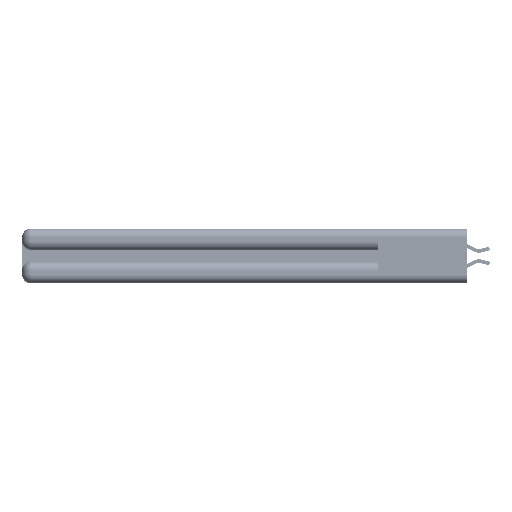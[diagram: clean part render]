
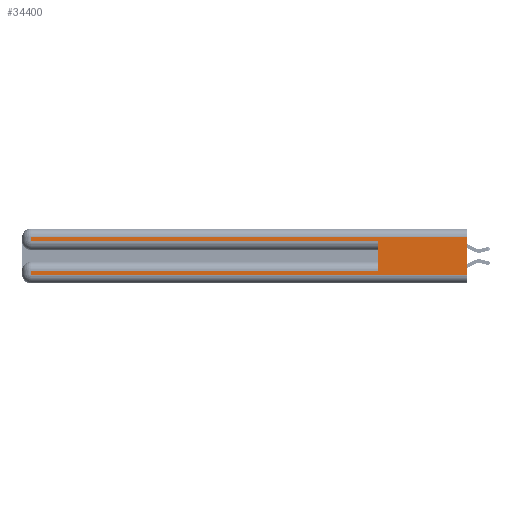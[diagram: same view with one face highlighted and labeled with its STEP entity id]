
A CAD part, left-side view. The second image highlights one B-rep face of the part: STEP entity #34400.
In plain terms, the highlighted planar face has unit normal (-1, 0, 0).
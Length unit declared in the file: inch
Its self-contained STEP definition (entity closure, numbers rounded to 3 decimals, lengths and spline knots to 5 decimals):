
#36 = CARTESIAN_POINT ( 'NONE',  ( 0., 2.94, 0.085 ) ) ;
#2518 = VERTEX_POINT ( 'NONE', #19276 ) ;
#2660 = CARTESIAN_POINT ( 'NONE',  ( 0., 2.94, 0.37 ) ) ;
#4139 = EDGE_CURVE ( 'NONE', #2518, #26555, #14256, .T. ) ;
#4845 = ORIENTED_EDGE ( 'NONE', *, *, #14804, .T. ) ;
#5372 = DIRECTION ( 'NONE',  ( 0., 1., 0. ) ) ;
#5791 = VECTOR ( 'NONE', #47952, 39.37008 ) ;
#6117 = VECTOR ( 'NONE', #49097, 39.37008 ) ;
#7320 = LINE ( 'NONE', #27149, #40049 ) ;
#8459 = ORIENTED_EDGE ( 'NONE', *, *, #17823, .F. ) ;
#8687 = CARTESIAN_POINT ( 'NONE',  ( 0., 2.94, 0.31 ) ) ;
#9255 = VERTEX_POINT ( 'NONE', #8687 ) ;
#11542 = VERTEX_POINT ( 'NONE', #28930 ) ;
#13489 = VERTEX_POINT ( 'NONE', #29145 ) ;
#14256 = LINE ( 'NONE', #31057, #48140 ) ;
#14804 = EDGE_CURVE ( 'NONE', #13489, #52597, #30994, .T. ) ;
#14828 = ORIENTED_EDGE ( 'NONE', *, *, #29586, .F. ) ;
#15429 = VECTOR ( 'NONE', #54866, 39.37008 ) ;
#15570 = FACE_OUTER_BOUND ( 'NONE', #28481, .T. ) ;
#16716 = CARTESIAN_POINT ( 'NONE',  ( 0., 0., 0.37 ) ) ;
#17246 = CARTESIAN_POINT ( 'NONE',  ( 0., 0.6, 0.285 ) ) ;
#17823 = EDGE_CURVE ( 'NONE', #11542, #31733, #49270, .T. ) ;
#18007 = VERTEX_POINT ( 'NONE', #25537 ) ;
#18516 = DIRECTION ( 'NONE',  ( 1., 0., 0. ) ) ;
#19276 = CARTESIAN_POINT ( 'NONE',  ( 0., 0.6, 0.085 ) ) ;
#19870 = CARTESIAN_POINT ( 'NONE',  ( 0., 0.6, 0.145 ) ) ;
#20956 = LINE ( 'NONE', #2660, #54731 ) ;
#22562 = CARTESIAN_POINT ( 'NONE',  ( 0., 0., 0.31 ) ) ;
#23254 = ORIENTED_EDGE ( 'NONE', *, *, #23889, .T. ) ;
#23721 = CARTESIAN_POINT ( 'NONE',  ( 0., 0., 0.06 ) ) ;
#23889 = EDGE_CURVE ( 'NONE', #18007, #31733, #28973, .T. ) ;
#24171 = CARTESIAN_POINT ( 'NONE',  ( 0., 0., 0.285 ) ) ;
#24805 = VECTOR ( 'NONE', #49502, 39.37008 ) ;
#25537 = CARTESIAN_POINT ( 'NONE',  ( 0., 2.94, 0.06 ) ) ;
#26409 = ORIENTED_EDGE ( 'NONE', *, *, #44551, .T. ) ;
#26555 = VERTEX_POINT ( 'NONE', #36 ) ;
#27149 = CARTESIAN_POINT ( 'NONE',  ( 0., 2.94, 0.37 ) ) ;
#28422 = DIRECTION ( 'NONE',  ( 0., 0., -1. ) ) ;
#28449 = DIRECTION ( 'NONE',  ( 0., -1., 0. ) ) ;
#28481 = EDGE_LOOP ( 'NONE', ( #8459, #37779, #26409, #4845, #14828, #51584, #37928, #23254 ) ) ;
#28930 = CARTESIAN_POINT ( 'NONE',  ( 0., 0., 0.31 ) ) ;
#28973 = LINE ( 'NONE', #23721, #6117 ) ;
#29145 = CARTESIAN_POINT ( 'NONE',  ( 0., 2.94, 0.285 ) ) ;
#29586 = EDGE_CURVE ( 'NONE', #2518, #52597, #40052, .T. ) ;
#30994 = LINE ( 'NONE', #24171, #42248 ) ;
#31057 = CARTESIAN_POINT ( 'NONE',  ( 0., 0., 0.085 ) ) ;
#31733 = VERTEX_POINT ( 'NONE', #53303 ) ;
#33109 = AXIS2_PLACEMENT_3D ( 'NONE', #43910, #18516, #48194 ) ;
#34400 = ADVANCED_FACE ( 'NONE', ( #15570 ), #35395, .F. ) ;
#35395 = PLANE ( 'NONE',  #33109 ) ;
#37779 = ORIENTED_EDGE ( 'NONE', *, *, #45996, .T. ) ;
#37928 = ORIENTED_EDGE ( 'NONE', *, *, #42946, .T. ) ;
#38560 = LINE ( 'NONE', #22562, #5791 ) ;
#40049 = VECTOR ( 'NONE', #44178, 39.37008 ) ;
#40052 = LINE ( 'NONE', #19870, #24805 ) ;
#42248 = VECTOR ( 'NONE', #28449, 39.37008 ) ;
#42946 = EDGE_CURVE ( 'NONE', #26555, #18007, #20956, .T. ) ;
#43910 = CARTESIAN_POINT ( 'NONE',  ( 0., 0., 0.37 ) ) ;
#44178 = DIRECTION ( 'NONE',  ( 0., 0., -1. ) ) ;
#44551 = EDGE_CURVE ( 'NONE', #9255, #13489, #7320, .T. ) ;
#45996 = EDGE_CURVE ( 'NONE', #11542, #9255, #38560, .T. ) ;
#47952 = DIRECTION ( 'NONE',  ( 0., 1., 0. ) ) ;
#48140 = VECTOR ( 'NONE', #5372, 39.37008 ) ;
#48194 = DIRECTION ( 'NONE',  ( 0., 0., -1. ) ) ;
#49097 = DIRECTION ( 'NONE',  ( 0., -1., 0. ) ) ;
#49270 = LINE ( 'NONE', #16716, #15429 ) ;
#49502 = DIRECTION ( 'NONE',  ( 0., 0., 1. ) ) ;
#51584 = ORIENTED_EDGE ( 'NONE', *, *, #4139, .T. ) ;
#52597 = VERTEX_POINT ( 'NONE', #17246 ) ;
#53303 = CARTESIAN_POINT ( 'NONE',  ( 0., 0., 0.06 ) ) ;
#54731 = VECTOR ( 'NONE', #28422, 39.37008 ) ;
#54866 = DIRECTION ( 'NONE',  ( 0., 0., -1. ) ) ;
